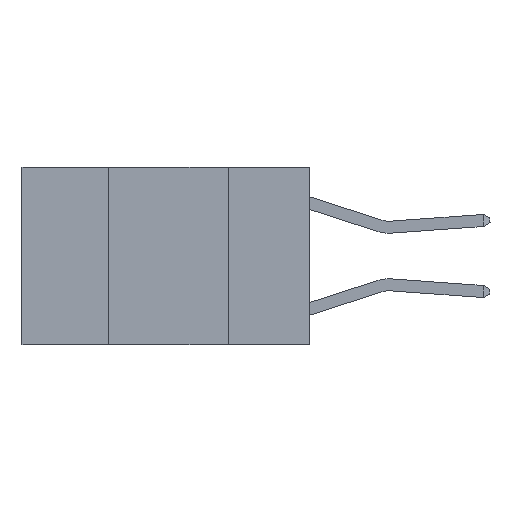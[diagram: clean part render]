
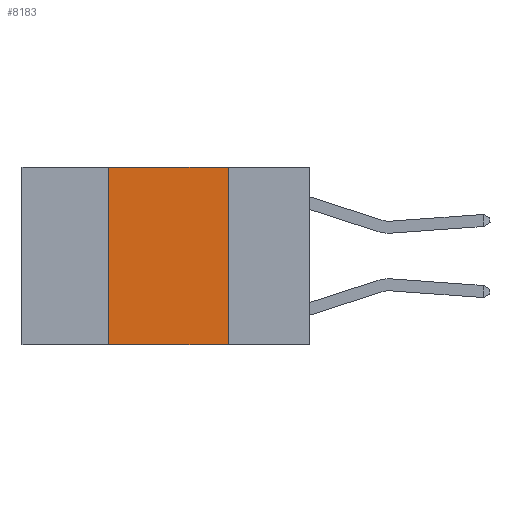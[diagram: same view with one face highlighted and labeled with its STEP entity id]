
A CAD part, left-side view. The second image highlights one B-rep face of the part: STEP entity #8183.
In plain terms, the highlighted planar face has unit normal (-1, 0, 0).
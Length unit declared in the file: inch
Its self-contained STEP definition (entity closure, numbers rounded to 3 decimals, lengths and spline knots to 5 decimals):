
#265 = AXIS2_PLACEMENT_3D ( 'NONE', #8478, #7719, #2391 ) ;
#1166 = VECTOR ( 'NONE', #3682, 39.37008 ) ;
#1817 = DIRECTION ( 'NONE',  ( 0., 0., 1. ) ) ;
#1880 = VERTEX_POINT ( 'NONE', #7336 ) ;
#1956 = FACE_OUTER_BOUND ( 'NONE', #3790, .T. ) ;
#2139 = ORIENTED_EDGE ( 'NONE', *, *, #6350, .T. ) ;
#2167 = DIRECTION ( 'NONE',  ( 0., 0., -1. ) ) ;
#2391 = DIRECTION ( 'NONE',  ( 0., 0., -1. ) ) ;
#2857 = ORIENTED_EDGE ( 'NONE', *, *, #6444, .F. ) ;
#2991 = VECTOR ( 'NONE', #7846, 39.37008 ) ;
#3277 = LINE ( 'NONE', #8655, #2991 ) ;
#3682 = DIRECTION ( 'NONE',  ( 0., -1., 0. ) ) ;
#3790 = EDGE_LOOP ( 'NONE', ( #9168, #2857, #6374, #2139 ) ) ;
#4023 = VERTEX_POINT ( 'NONE', #7157 ) ;
#4147 = VECTOR ( 'NONE', #1817, 39.37008 ) ;
#4605 = LINE ( 'NONE', #9851, #10818 ) ;
#6037 = PLANE ( 'NONE',  #265 ) ;
#6114 = CARTESIAN_POINT ( 'NONE',  ( 0., 0.17, -0.37 ) ) ;
#6350 = EDGE_CURVE ( 'NONE', #4023, #8256, #3277, .T. ) ;
#6374 = ORIENTED_EDGE ( 'NONE', *, *, #6860, .F. ) ;
#6444 = EDGE_CURVE ( 'NONE', #1880, #10384, #10374, .T. ) ;
#6860 = EDGE_CURVE ( 'NONE', #4023, #1880, #7033, .T. ) ;
#7033 = LINE ( 'NONE', #9599, #4147 ) ;
#7157 = CARTESIAN_POINT ( 'NONE',  ( 0., 0.42, -0.37 ) ) ;
#7336 = CARTESIAN_POINT ( 'NONE',  ( 0., 0.42, 0. ) ) ;
#7719 = DIRECTION ( 'NONE',  ( 1., 0., 0. ) ) ;
#7846 = DIRECTION ( 'NONE',  ( 0., -1., 0. ) ) ;
#7967 = EDGE_CURVE ( 'NONE', #10384, #8256, #4605, .T. ) ;
#8183 = ADVANCED_FACE ( 'NONE', ( #1956 ), #6037, .F. ) ;
#8256 = VERTEX_POINT ( 'NONE', #6114 ) ;
#8478 = CARTESIAN_POINT ( 'NONE',  ( 0., 0.6, 0. ) ) ;
#8655 = CARTESIAN_POINT ( 'NONE',  ( 0., 0.6, -0.37 ) ) ;
#9168 = ORIENTED_EDGE ( 'NONE', *, *, #7967, .F. ) ;
#9599 = CARTESIAN_POINT ( 'NONE',  ( 0., 0.42, 0. ) ) ;
#9851 = CARTESIAN_POINT ( 'NONE',  ( 0., 0.17, 0. ) ) ;
#10125 = CARTESIAN_POINT ( 'NONE',  ( 0., 0.17, 0. ) ) ;
#10374 = LINE ( 'NONE', #11143, #1166 ) ;
#10384 = VERTEX_POINT ( 'NONE', #10125 ) ;
#10818 = VECTOR ( 'NONE', #2167, 39.37008 ) ;
#11143 = CARTESIAN_POINT ( 'NONE',  ( 0., 0.6, 0. ) ) ;
